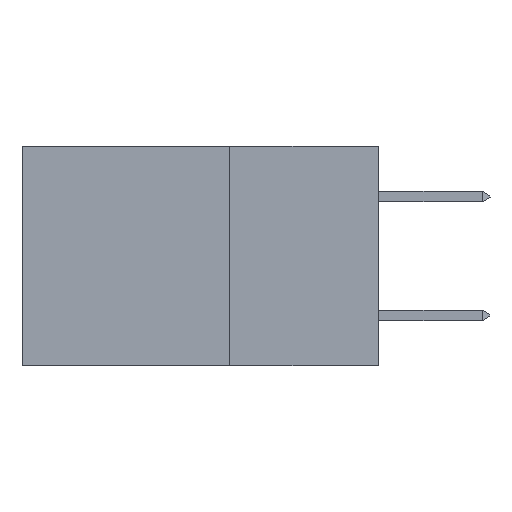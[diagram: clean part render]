
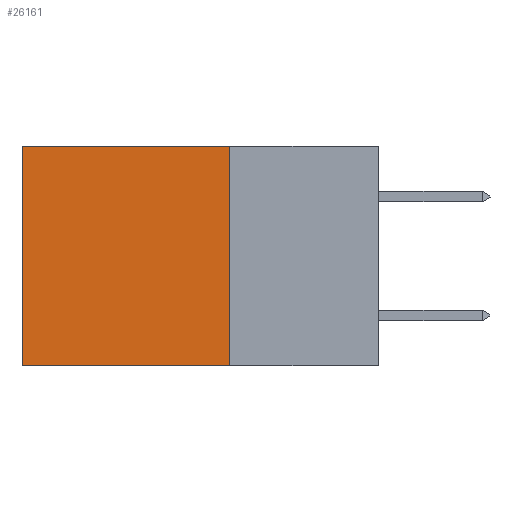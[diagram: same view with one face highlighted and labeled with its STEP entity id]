
A CAD part, left-side view. The second image highlights one B-rep face of the part: STEP entity #26161.
In plain terms, the highlighted planar face has unit normal (-1, 0, 0).
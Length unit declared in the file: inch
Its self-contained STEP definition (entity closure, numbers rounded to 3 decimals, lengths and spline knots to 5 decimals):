
#733 = FACE_OUTER_BOUND ( 'NONE', #33089, .T. ) ;
#2737 = DIRECTION ( 'NONE',  ( 1., 0., 0. ) ) ;
#3072 = PLANE ( 'NONE',  #27279 ) ;
#3507 = ORIENTED_EDGE ( 'NONE', *, *, #6890, .T. ) ;
#3666 = ORIENTED_EDGE ( 'NONE', *, *, #23640, .F. ) ;
#4277 = CARTESIAN_POINT ( 'NONE',  ( 0.298, 0.6, -0.37 ) ) ;
#5601 = DIRECTION ( 'NONE',  ( 0., 0., -1. ) ) ;
#6890 = EDGE_CURVE ( 'NONE', #29893, #32165, #12921, .T. ) ;
#7500 = CARTESIAN_POINT ( 'NONE',  ( 0.298, 0.25, 0. ) ) ;
#8021 = CARTESIAN_POINT ( 'NONE',  ( 0.298, 0.25, 0. ) ) ;
#8541 = VERTEX_POINT ( 'NONE', #7500 ) ;
#8985 = VECTOR ( 'NONE', #9268, 39.37008 ) ;
#9268 = DIRECTION ( 'NONE',  ( 0., 1., 0. ) ) ;
#9732 = CARTESIAN_POINT ( 'NONE',  ( 0.298, 0.25, 0. ) ) ;
#11198 = VERTEX_POINT ( 'NONE', #24619 ) ;
#12921 = LINE ( 'NONE', #28793, #32554 ) ;
#12961 = LINE ( 'NONE', #8021, #14154 ) ;
#14154 = VECTOR ( 'NONE', #25948, 39.37008 ) ;
#18427 = EDGE_CURVE ( 'NONE', #8541, #29893, #25357, .T. ) ;
#20024 = CARTESIAN_POINT ( 'NONE',  ( 0.298, 0.25, -0.37 ) ) ;
#20612 = DIRECTION ( 'NONE',  ( 0., 1., 0. ) ) ;
#20723 = DIRECTION ( 'NONE',  ( 0., 0., -1. ) ) ;
#23640 = EDGE_CURVE ( 'NONE', #11198, #32165, #30207, .T. ) ;
#23920 = EDGE_CURVE ( 'NONE', #8541, #11198, #12961, .T. ) ;
#24619 = CARTESIAN_POINT ( 'NONE',  ( 0.298, 0.25, -0.37 ) ) ;
#25357 = LINE ( 'NONE', #9732, #26925 ) ;
#25948 = DIRECTION ( 'NONE',  ( 0., 0., -1. ) ) ;
#26082 = CARTESIAN_POINT ( 'NONE',  ( 0.298, 0.25, 0. ) ) ;
#26161 = ADVANCED_FACE ( 'NONE', ( #733 ), #3072, .F. ) ;
#26925 = VECTOR ( 'NONE', #20612, 39.37008 ) ;
#27279 = AXIS2_PLACEMENT_3D ( 'NONE', #26082, #2737, #20723 ) ;
#27562 = ORIENTED_EDGE ( 'NONE', *, *, #23920, .F. ) ;
#28793 = CARTESIAN_POINT ( 'NONE',  ( 0.298, 0.6, 0. ) ) ;
#29893 = VERTEX_POINT ( 'NONE', #32644 ) ;
#30207 = LINE ( 'NONE', #20024, #8985 ) ;
#30622 = ORIENTED_EDGE ( 'NONE', *, *, #18427, .T. ) ;
#32165 = VERTEX_POINT ( 'NONE', #4277 ) ;
#32554 = VECTOR ( 'NONE', #5601, 39.37008 ) ;
#32644 = CARTESIAN_POINT ( 'NONE',  ( 0.298, 0.6, 0. ) ) ;
#33089 = EDGE_LOOP ( 'NONE', ( #3507, #3666, #27562, #30622 ) ) ;
